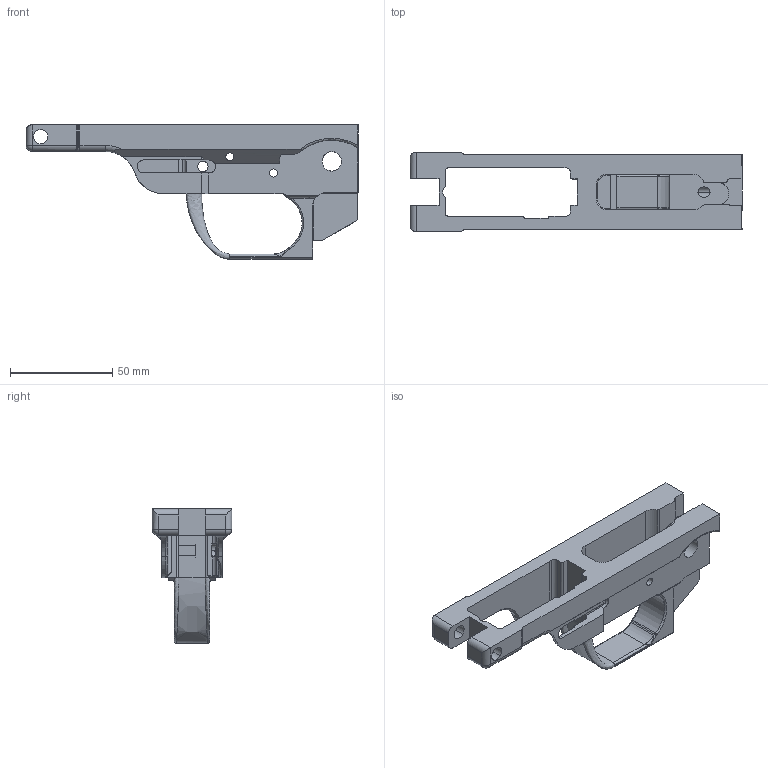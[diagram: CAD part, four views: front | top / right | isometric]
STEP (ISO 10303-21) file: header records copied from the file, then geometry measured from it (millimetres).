
FILE_DESCRIPTION (( 'STEP AP214' ), '1' );
FILE_NAME ('Phobos_V1.2_Front.STEP', '2015-05-21T06:10:34', ( 'WarFairy' ), ( '' ), 'SwSTEP 2.0', 'SolidWorks 2015', '' );
FILE_SCHEMA (( 'AUTOMOTIVE_DESIGN' ));
Length unit declared in the file: inch
Products named in the file (1): Phobos_V1.2_Front
Bounding box: 162.67 x 39 x 65.79 mm (x, y, z)
Volume: 75177 mm3; surface area: 33165.3 mm2
Topology: 1 solids, 1 shells, 282 faces, 798 edges, 503 vertices
Faces by surface type: cylinder 118, plane 96, bspline 29, torus 21, cone 15, sphere 3
Entity records: 13060 total; most frequent: CARTESIAN_POINT 6023, ORIENTED_EDGE 1584, DIRECTION 1322, EDGE_CURVE 792, VERTEX_POINT 503, AXIS2_PLACEMENT_3D 462, VECTOR 398, LINE 398
